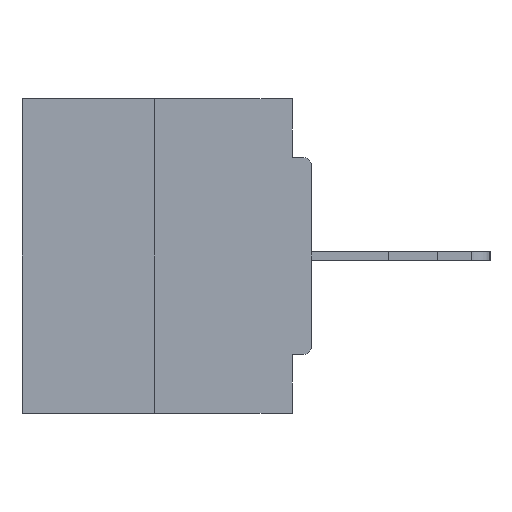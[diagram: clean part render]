
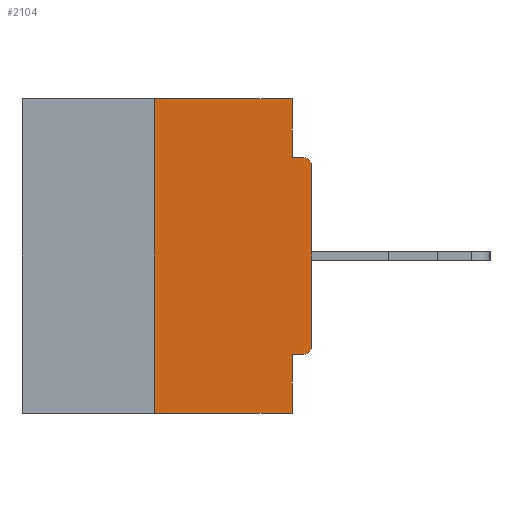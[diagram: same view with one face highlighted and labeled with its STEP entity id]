
A CAD part, left-side view. The second image highlights one B-rep face of the part: STEP entity #2104.
In plain terms, the highlighted planar face has unit normal (-1, 0, 0).
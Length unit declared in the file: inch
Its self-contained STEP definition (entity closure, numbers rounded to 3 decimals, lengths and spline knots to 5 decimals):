
#627 = AXIS2_PLACEMENT_3D ( 'NONE', #18250, #4453, #20503 ) ;
#823 = ORIENTED_EDGE ( 'NONE', *, *, #14321, .F. ) ;
#1158 = CIRCLE ( 'NONE', #5838, 0.015 ) ;
#1185 = ORIENTED_EDGE ( 'NONE', *, *, #23452, .F. ) ;
#1795 = CARTESIAN_POINT ( 'NONE',  ( 0., 0.031, -0.4065 ) ) ;
#2104 = ADVANCED_FACE ( 'NONE', ( #10284 ), #15399, .F. ) ;
#2290 = CARTESIAN_POINT ( 'NONE',  ( 0., 0.25, 0. ) ) ;
#3158 = CARTESIAN_POINT ( 'NONE',  ( 0., 0.031, -0.5 ) ) ;
#3477 = EDGE_CURVE ( 'NONE', #11454, #18141, #1158, .T. ) ;
#3543 = VECTOR ( 'NONE', #7072, 39.37008 ) ;
#3751 = VERTEX_POINT ( 'NONE', #1795 ) ;
#3864 = CARTESIAN_POINT ( 'NONE',  ( 0., 0., -0.0935 ) ) ;
#3954 = VERTEX_POINT ( 'NONE', #10648 ) ;
#4293 = LINE ( 'NONE', #2290, #3543 ) ;
#4453 = DIRECTION ( 'NONE',  ( -1., 0., 0. ) ) ;
#4621 = VERTEX_POINT ( 'NONE', #23270 ) ;
#5118 = CARTESIAN_POINT ( 'NONE',  ( 0., 0., -0.4065 ) ) ;
#5188 = ORIENTED_EDGE ( 'NONE', *, *, #15473, .F. ) ;
#5838 = AXIS2_PLACEMENT_3D ( 'NONE', #21699, #21691, #16455 ) ;
#7072 = DIRECTION ( 'NONE',  ( 0., 0., 1. ) ) ;
#7364 = VECTOR ( 'NONE', #9222, 39.37008 ) ;
#7450 = DIRECTION ( 'NONE',  ( 0., 1., 0. ) ) ;
#8097 = LINE ( 'NONE', #16064, #7364 ) ;
#8102 = ORIENTED_EDGE ( 'NONE', *, *, #8173, .T. ) ;
#8173 = EDGE_CURVE ( 'NONE', #3954, #11373, #13354, .T. ) ;
#9005 = EDGE_CURVE ( 'NONE', #25045, #29083, #14024, .T. ) ;
#9222 = DIRECTION ( 'NONE',  ( 0., 0., 1. ) ) ;
#9303 = EDGE_CURVE ( 'NONE', #29083, #16728, #28913, .T. ) ;
#9736 = CARTESIAN_POINT ( 'NONE',  ( 0., 0.46, 0. ) ) ;
#10284 = FACE_OUTER_BOUND ( 'NONE', #14057, .T. ) ;
#10648 = CARTESIAN_POINT ( 'NONE',  ( 0., 0.015, -0.4065 ) ) ;
#10814 = DIRECTION ( 'NONE',  ( 0., 0., -1. ) ) ;
#10828 = EDGE_CURVE ( 'NONE', #3751, #4621, #18655, .T. ) ;
#11373 = VERTEX_POINT ( 'NONE', #11921 ) ;
#11454 = VERTEX_POINT ( 'NONE', #14634 ) ;
#11921 = CARTESIAN_POINT ( 'NONE',  ( 0., 0., -0.3915 ) ) ;
#12371 = EDGE_CURVE ( 'NONE', #15941, #4621, #14242, .T. ) ;
#12735 = ORIENTED_EDGE ( 'NONE', *, *, #10828, .F. ) ;
#13007 = VECTOR ( 'NONE', #28946, 39.37008 ) ;
#13354 = CIRCLE ( 'NONE', #627, 0.015 ) ;
#13360 = CARTESIAN_POINT ( 'NONE',  ( 0., 0.25, -0.5 ) ) ;
#13485 = CARTESIAN_POINT ( 'NONE',  ( 0., 0.25, 0. ) ) ;
#13507 = VECTOR ( 'NONE', #18021, 39.37008 ) ;
#13740 = LINE ( 'NONE', #3864, #13007 ) ;
#14024 = LINE ( 'NONE', #9736, #24701 ) ;
#14057 = EDGE_LOOP ( 'NONE', ( #16724, #5188, #18165, #12735, #1185, #8102, #27009, #21688, #823, #25234 ) ) ;
#14242 = LINE ( 'NONE', #22546, #13507 ) ;
#14321 = EDGE_CURVE ( 'NONE', #16728, #18141, #13740, .T. ) ;
#14468 = CARTESIAN_POINT ( 'NONE',  ( 0., 0.031, 0. ) ) ;
#14634 = CARTESIAN_POINT ( 'NONE',  ( 0., 0., -0.1085 ) ) ;
#15399 = PLANE ( 'NONE',  #22478 ) ;
#15473 = EDGE_CURVE ( 'NONE', #15941, #25045, #4293, .T. ) ;
#15941 = VERTEX_POINT ( 'NONE', #13360 ) ;
#16064 = CARTESIAN_POINT ( 'NONE',  ( 0., 0., 0. ) ) ;
#16163 = VECTOR ( 'NONE', #10814, 39.37008 ) ;
#16455 = DIRECTION ( 'NONE',  ( 0., 0., -1. ) ) ;
#16589 = CARTESIAN_POINT ( 'NONE',  ( 0., 0.46, 0. ) ) ;
#16724 = ORIENTED_EDGE ( 'NONE', *, *, #9005, .F. ) ;
#16728 = VERTEX_POINT ( 'NONE', #18463 ) ;
#17084 = CARTESIAN_POINT ( 'NONE',  ( 0., 0.015, -0.0935 ) ) ;
#17932 = VECTOR ( 'NONE', #23806, 39.37008 ) ;
#18021 = DIRECTION ( 'NONE',  ( 0., -1., 0. ) ) ;
#18141 = VERTEX_POINT ( 'NONE', #17084 ) ;
#18165 = ORIENTED_EDGE ( 'NONE', *, *, #12371, .T. ) ;
#18250 = CARTESIAN_POINT ( 'NONE',  ( 0., 0.015, -0.3915 ) ) ;
#18463 = CARTESIAN_POINT ( 'NONE',  ( 0., 0.031, -0.0935 ) ) ;
#18655 = LINE ( 'NONE', #3158, #17932 ) ;
#20419 = DIRECTION ( 'NONE',  ( 1., 0., 0. ) ) ;
#20503 = DIRECTION ( 'NONE',  ( 0., 0., -1. ) ) ;
#21219 = DIRECTION ( 'NONE',  ( 0., -1., 0. ) ) ;
#21246 = DIRECTION ( 'NONE',  ( 0., 0., -1. ) ) ;
#21688 = ORIENTED_EDGE ( 'NONE', *, *, #3477, .T. ) ;
#21691 = DIRECTION ( 'NONE',  ( -1., 0., 0. ) ) ;
#21699 = CARTESIAN_POINT ( 'NONE',  ( 0., 0.015, -0.1085 ) ) ;
#22478 = AXIS2_PLACEMENT_3D ( 'NONE', #16589, #20419, #21246 ) ;
#22546 = CARTESIAN_POINT ( 'NONE',  ( 0., 0.46, -0.5 ) ) ;
#23270 = CARTESIAN_POINT ( 'NONE',  ( 0., 0.031, -0.5 ) ) ;
#23452 = EDGE_CURVE ( 'NONE', #3954, #3751, #24390, .T. ) ;
#23806 = DIRECTION ( 'NONE',  ( 0., 0., -1. ) ) ;
#24385 = CARTESIAN_POINT ( 'NONE',  ( 0., 0.031, 0. ) ) ;
#24390 = LINE ( 'NONE', #5118, #28990 ) ;
#24701 = VECTOR ( 'NONE', #21219, 39.37008 ) ;
#25045 = VERTEX_POINT ( 'NONE', #13485 ) ;
#25234 = ORIENTED_EDGE ( 'NONE', *, *, #9303, .F. ) ;
#27009 = ORIENTED_EDGE ( 'NONE', *, *, #29531, .T. ) ;
#28913 = LINE ( 'NONE', #24385, #16163 ) ;
#28946 = DIRECTION ( 'NONE',  ( 0., -1., 0. ) ) ;
#28990 = VECTOR ( 'NONE', #7450, 39.37008 ) ;
#29083 = VERTEX_POINT ( 'NONE', #14468 ) ;
#29531 = EDGE_CURVE ( 'NONE', #11373, #11454, #8097, .T. ) ;
